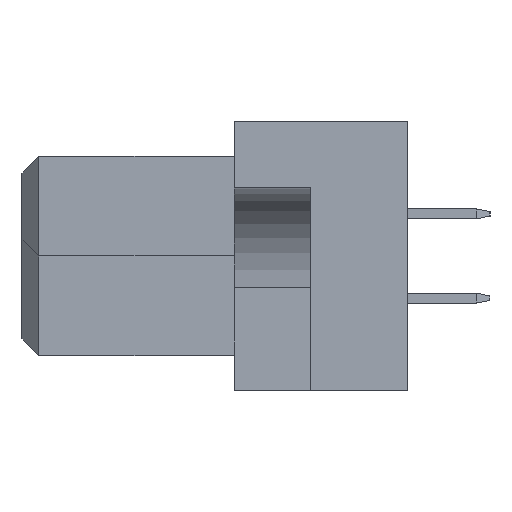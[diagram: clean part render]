
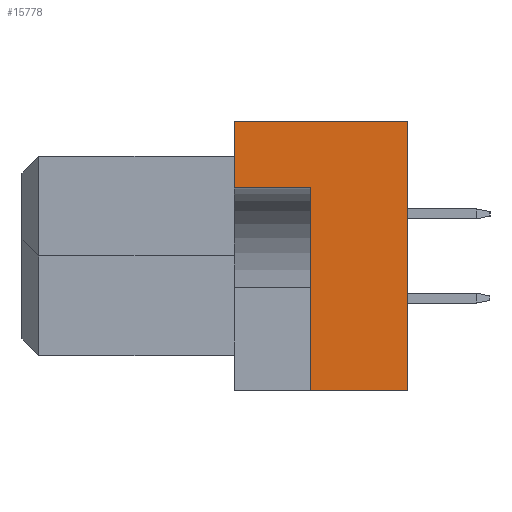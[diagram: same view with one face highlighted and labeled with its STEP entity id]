
A CAD part, left-side view. The second image highlights one B-rep face of the part: STEP entity #15778.
In plain terms, the highlighted planar face has unit normal (-1, 0, 0).
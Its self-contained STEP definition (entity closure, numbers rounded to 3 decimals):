
#989 = VERTEX_POINT ( 'NONE', #6528 ) ;
#1340 = DIRECTION ( 'NONE',  ( 0., -1., 0. ) ) ;
#1506 = VECTOR ( 'NONE', #1340, 1000. ) ;
#1753 = ORIENTED_EDGE ( 'NONE', *, *, #14509, .F. ) ;
#1820 = VERTEX_POINT ( 'NONE', #13897 ) ;
#1913 = ORIENTED_EDGE ( 'NONE', *, *, #6853, .F. ) ;
#2809 = DIRECTION ( 'NONE',  ( 0., 0., 1. ) ) ;
#3454 = DIRECTION ( 'NONE',  ( 0., 0., -1. ) ) ;
#3643 = EDGE_CURVE ( 'NONE', #10639, #12994, #7320, .T. ) ;
#3823 = ORIENTED_EDGE ( 'NONE', *, *, #13899, .T. ) ;
#3829 = CARTESIAN_POINT ( 'NONE',  ( -35.12, 5.2, -4.05 ) ) ;
#3893 = CARTESIAN_POINT ( 'NONE',  ( -35.12, 2.9, 2.05 ) ) ;
#5694 = CARTESIAN_POINT ( 'NONE',  ( -35.12, 0., -4.05 ) ) ;
#5695 = CARTESIAN_POINT ( 'NONE',  ( -35.12, 5.2, 4.05 ) ) ;
#5844 = DIRECTION ( 'NONE',  ( 0., 0., 1. ) ) ;
#5899 = CARTESIAN_POINT ( 'NONE',  ( -35.12, 2.9, 2.05 ) ) ;
#5908 = VECTOR ( 'NONE', #5844, 1000. ) ;
#6528 = CARTESIAN_POINT ( 'NONE',  ( -35.12, 5.2, 4.05 ) ) ;
#6853 = EDGE_CURVE ( 'NONE', #1820, #989, #9963, .T. ) ;
#7320 = LINE ( 'NONE', #13385, #5908 ) ;
#7555 = LINE ( 'NONE', #19546, #16696 ) ;
#7768 = VECTOR ( 'NONE', #8528, 1000. ) ;
#7913 = EDGE_CURVE ( 'NONE', #17627, #1820, #11704, .T. ) ;
#8528 = DIRECTION ( 'NONE',  ( 0., 1., 0. ) ) ;
#9789 = ORIENTED_EDGE ( 'NONE', *, *, #3643, .T. ) ;
#9963 = LINE ( 'NONE', #11344, #19386 ) ;
#10639 = VERTEX_POINT ( 'NONE', #5694 ) ;
#11011 = CARTESIAN_POINT ( 'NONE',  ( -35.12, 0., 4.05 ) ) ;
#11344 = CARTESIAN_POINT ( 'NONE',  ( -35.12, 5.2, 4.05 ) ) ;
#11704 = LINE ( 'NONE', #3893, #7768 ) ;
#12994 = VERTEX_POINT ( 'NONE', #11011 ) ;
#13138 = FACE_OUTER_BOUND ( 'NONE', #13192, .T. ) ;
#13192 = EDGE_LOOP ( 'NONE', ( #1913, #18043, #1753, #3823, #9789, #17795 ) ) ;
#13385 = CARTESIAN_POINT ( 'NONE',  ( -35.12, 0., 4.05 ) ) ;
#13546 = VECTOR ( 'NONE', #17506, 1000. ) ;
#13897 = CARTESIAN_POINT ( 'NONE',  ( -35.12, 5.2, 2.05 ) ) ;
#13899 = EDGE_CURVE ( 'NONE', #19359, #10639, #19187, .T. ) ;
#14110 = EDGE_CURVE ( 'NONE', #989, #12994, #14918, .T. ) ;
#14509 = EDGE_CURVE ( 'NONE', #19359, #17627, #7555, .T. ) ;
#14918 = LINE ( 'NONE', #16407, #1506 ) ;
#15365 = CARTESIAN_POINT ( 'NONE',  ( -35.12, 2.9, -4.05 ) ) ;
#15536 = PLANE ( 'NONE',  #18095 ) ;
#15778 = ADVANCED_FACE ( 'NONE', ( #13138 ), #15536, .F. ) ;
#16407 = CARTESIAN_POINT ( 'NONE',  ( -35.12, 5.2, 4.05 ) ) ;
#16696 = VECTOR ( 'NONE', #2809, 1000. ) ;
#17020 = DIRECTION ( 'NONE',  ( 1., 0., 0. ) ) ;
#17498 = DIRECTION ( 'NONE',  ( 0., 0., 1. ) ) ;
#17506 = DIRECTION ( 'NONE',  ( 0., -1., 0. ) ) ;
#17627 = VERTEX_POINT ( 'NONE', #5899 ) ;
#17795 = ORIENTED_EDGE ( 'NONE', *, *, #14110, .F. ) ;
#18043 = ORIENTED_EDGE ( 'NONE', *, *, #7913, .F. ) ;
#18095 = AXIS2_PLACEMENT_3D ( 'NONE', #5695, #17020, #3454 ) ;
#19187 = LINE ( 'NONE', #3829, #13546 ) ;
#19359 = VERTEX_POINT ( 'NONE', #15365 ) ;
#19386 = VECTOR ( 'NONE', #17498, 1000. ) ;
#19546 = CARTESIAN_POINT ( 'NONE',  ( -35.12, 2.9, 2.05 ) ) ;
